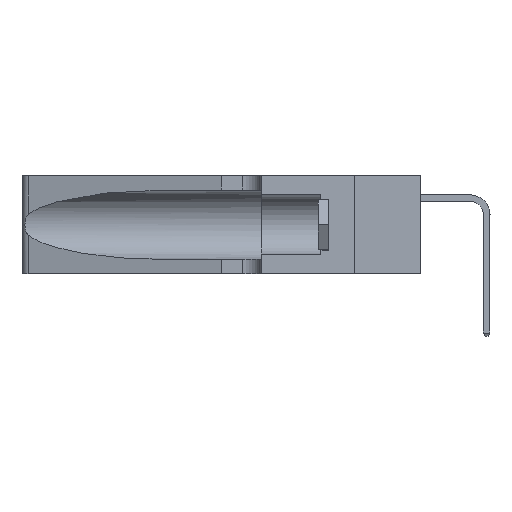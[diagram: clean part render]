
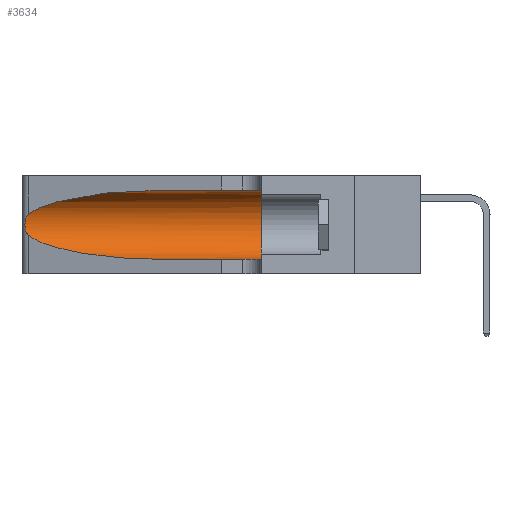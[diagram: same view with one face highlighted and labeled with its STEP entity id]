
A CAD part, left-side view. The second image highlights one B-rep face of the part: STEP entity #3634.
In plain terms, the highlighted cylindrical face has radius 3.308 mm (diameter 6.617 mm), a partial arc.
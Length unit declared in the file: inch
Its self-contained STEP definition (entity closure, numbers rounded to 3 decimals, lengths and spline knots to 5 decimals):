
#220 = EDGE_CURVE ( 'NONE', #20804, #19937, #21835, .T. ) ;
#933 = CARTESIAN_POINT ( 'NONE',  ( 0.26075, 1.23896, 0.19203 ) ) ;
#1495 = LINE ( 'NONE', #37508, #15481 ) ;
#3400 = EDGE_CURVE ( 'NONE', #22219, #7537, #33406, .T. ) ;
#3634 = ADVANCED_FACE ( 'NONE', ( #25424 ), #14939, .F. ) ;
#4169 = CARTESIAN_POINT ( 'NONE',  ( 0.26017, 1.23833, 0.17102 ) ) ;
#4303 = CARTESIAN_POINT ( 'NONE',  ( 0.1305, 0.35, 0.31525 ) ) ;
#5435 = CARTESIAN_POINT ( 'NONE',  ( 0.1305, 1.61858, 0.05475 ) ) ;
#5527 = CARTESIAN_POINT ( 'NONE',  ( 0.25487, 1.22718, 0.22369 ) ) ;
#6441 = AXIS2_PLACEMENT_3D ( 'NONE', #14377, #36638, #17591 ) ;
#7390 = CARTESIAN_POINT ( 'NONE',  ( 0.25789, 1.23486, 0.15765 ) ) ;
#7537 = VERTEX_POINT ( 'NONE', #37124 ) ;
#9936 = AXIS2_PLACEMENT_3D ( 'NONE', #31457, #18693, #12396 ) ;
#10467 = CARTESIAN_POINT ( 'NONE',  ( 0.25487, 1.22718, 0.22369 ) ) ;
#10598 = CARTESIAN_POINT ( 'NONE',  ( 0.25555, 1.22993, 0.14849 ) ) ;
#12396 = DIRECTION ( 'NONE',  ( 0., 0., -1. ) ) ;
#12648 = CARTESIAN_POINT ( 'NONE',  ( 0.25487, 1.22718, 0.14631 ) ) ;
#13507 =( BOUNDED_CURVE ( )  B_SPLINE_CURVE ( 3, ( #35196, #31961, #38344, #19318 ),
 .UNSPECIFIED., .F., .T. ) 
 B_SPLINE_CURVE_WITH_KNOTS ( ( 4, 4 ),
 ( 1.5708, 2.84003 ),
 .UNSPECIFIED. ) 
 CURVE ( )  GEOMETRIC_REPRESENTATION_ITEM ( )  RATIONAL_B_SPLINE_CURVE ( ( 1., 0.87, 0.87, 1. ) ) 
 REPRESENTATION_ITEM ( '' )  );
#13509 = ORIENTED_EDGE ( 'NONE', *, *, #3400, .F. ) ;
#14377 = CARTESIAN_POINT ( 'NONE',  ( 0.1305, 0.35, 0.185 ) ) ;
#14939 = CYLINDRICAL_SURFACE ( 'NONE', #9936, 0.13025 ) ;
#15344 = ORIENTED_EDGE ( 'NONE', *, *, #22668, .T. ) ;
#15481 = VECTOR ( 'NONE', #34367, 39.37008 ) ;
#16863 = CARTESIAN_POINT ( 'NONE',  ( 0.25787, 1.23484, 0.2124 ) ) ;
#17591 = DIRECTION ( 'NONE',  ( 0., 0., 1. ) ) ;
#18693 = DIRECTION ( 'NONE',  ( 0., -1., 0. ) ) ;
#19318 = CARTESIAN_POINT ( 'NONE',  ( 0.25487, 1.22718, 0.22369 ) ) ;
#19469 = VERTEX_POINT ( 'NONE', #5527 ) ;
#19519 = EDGE_CURVE ( 'NONE', #38609, #22219, #1495, .T. ) ;
#19937 = VERTEX_POINT ( 'NONE', #33785 ) ;
#20071 = CARTESIAN_POINT ( 'NONE',  ( 0.26018, 1.23835, 0.19895 ) ) ;
#20804 = VERTEX_POINT ( 'NONE', #28680 ) ;
#21835 =( BOUNDED_CURVE ( )  B_SPLINE_CURVE ( 3, ( #12648, #40614, #31310, #28665 ),
 .UNSPECIFIED., .F., .F. ) 
 B_SPLINE_CURVE_WITH_KNOTS ( ( 4, 4 ),
 ( 3.44316, 4.71239 ),
 .UNSPECIFIED. ) 
 CURVE ( )  GEOMETRIC_REPRESENTATION_ITEM ( )  RATIONAL_B_SPLINE_CURVE ( ( 1., 0.87, 0.87, 1. ) ) 
 REPRESENTATION_ITEM ( '' )  );
#22219 = VERTEX_POINT ( 'NONE', #4303 ) ;
#22520 = LINE ( 'NONE', #5435, #30961 ) ;
#22668 = EDGE_CURVE ( 'NONE', #38609, #19469, #13507, .T. ) ;
#23118 = B_SPLINE_CURVE_WITH_KNOTS ( 'NONE', 3,
 ( #10467, #29527, #35916, #16863, #39107, #20071, #933, #23273, #4169, #26463, #7390, #29670, #10598, #32878 ),
 .UNSPECIFIED., .F., .F.,
 ( 4, 2, 2, 2, 2, 2, 4 ),
 ( 0., 0.00027, 0.00053, 0.00107, 0.0016, 0.00187, 0.00214 ),
 .UNSPECIFIED. ) ;
#23273 = CARTESIAN_POINT ( 'NONE',  ( 0.26075, 1.23896, 0.178 ) ) ;
#24507 = ORIENTED_EDGE ( 'NONE', *, *, #39396, .T. ) ;
#24834 = ORIENTED_EDGE ( 'NONE', *, *, #30101, .T. ) ;
#25424 = FACE_OUTER_BOUND ( 'NONE', #35709, .T. ) ;
#26463 = CARTESIAN_POINT ( 'NONE',  ( 0.25856, 1.23593, 0.16098 ) ) ;
#27711 = DIRECTION ( 'NONE',  ( 0., -1., 0. ) ) ;
#28665 = CARTESIAN_POINT ( 'NONE',  ( 0.1305, 0.72297, 0.05475 ) ) ;
#28680 = CARTESIAN_POINT ( 'NONE',  ( 0.25487, 1.22718, 0.14631 ) ) ;
#29527 = CARTESIAN_POINT ( 'NONE',  ( 0.25555, 1.22994, 0.2215 ) ) ;
#29670 = CARTESIAN_POINT ( 'NONE',  ( 0.25639, 1.23186, 0.15144 ) ) ;
#30101 = EDGE_CURVE ( 'NONE', #19469, #20804, #23118, .T. ) ;
#30961 = VECTOR ( 'NONE', #27711, 39.37008 ) ;
#31310 = CARTESIAN_POINT ( 'NONE',  ( 0.18966, 0.96281, 0.05475 ) ) ;
#31457 = CARTESIAN_POINT ( 'NONE',  ( 0.1305, 1.61858, 0.185 ) ) ;
#31961 = CARTESIAN_POINT ( 'NONE',  ( 0.18966, 0.96281, 0.31525 ) ) ;
#32878 = CARTESIAN_POINT ( 'NONE',  ( 0.25487, 1.22718, 0.14631 ) ) ;
#33406 = CIRCLE ( 'NONE', #6441, 0.13025 ) ;
#33785 = CARTESIAN_POINT ( 'NONE',  ( 0.1305, 0.72297, 0.05475 ) ) ;
#34367 = DIRECTION ( 'NONE',  ( 0., -1., 0. ) ) ;
#35196 = CARTESIAN_POINT ( 'NONE',  ( 0.1305, 0.72297, 0.31525 ) ) ;
#35709 = EDGE_LOOP ( 'NONE', ( #15344, #24834, #36960, #24507, #13509, #40886 ) ) ;
#35916 = CARTESIAN_POINT ( 'NONE',  ( 0.25639, 1.23184, 0.21858 ) ) ;
#36638 = DIRECTION ( 'NONE',  ( 0., 1., 0. ) ) ;
#36960 = ORIENTED_EDGE ( 'NONE', *, *, #220, .T. ) ;
#37124 = CARTESIAN_POINT ( 'NONE',  ( 0.1305, 0.35, 0.05475 ) ) ;
#37508 = CARTESIAN_POINT ( 'NONE',  ( 0.1305, 1.61858, 0.31525 ) ) ;
#38344 = CARTESIAN_POINT ( 'NONE',  ( 0.2373, 1.15595, 0.28018 ) ) ;
#38609 = VERTEX_POINT ( 'NONE', #39333 ) ;
#39107 = CARTESIAN_POINT ( 'NONE',  ( 0.25854, 1.2359, 0.20912 ) ) ;
#39333 = CARTESIAN_POINT ( 'NONE',  ( 0.1305, 0.72297, 0.31525 ) ) ;
#39396 = EDGE_CURVE ( 'NONE', #19937, #7537, #22520, .T. ) ;
#40614 = CARTESIAN_POINT ( 'NONE',  ( 0.2373, 1.15595, 0.08982 ) ) ;
#40886 = ORIENTED_EDGE ( 'NONE', *, *, #19519, .F. ) ;
